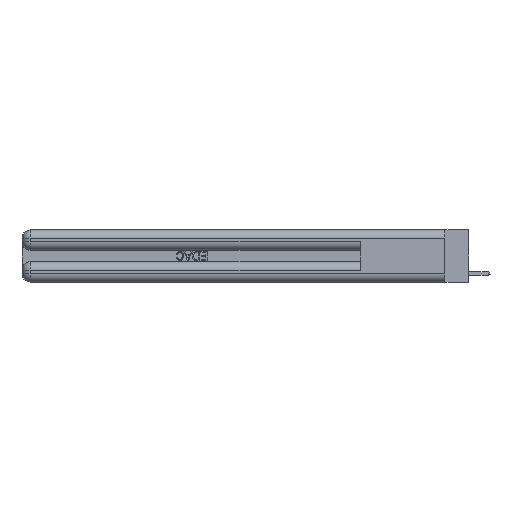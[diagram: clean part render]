
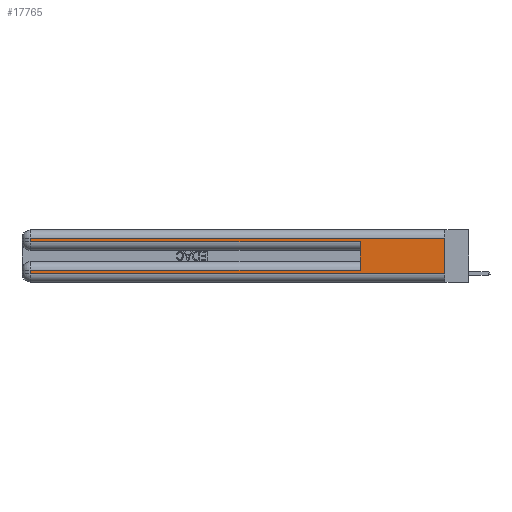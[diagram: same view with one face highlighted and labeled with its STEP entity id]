
A CAD part, left-side view. The second image highlights one B-rep face of the part: STEP entity #17765.
In plain terms, the highlighted planar face has unit normal (-1, 0, 0).
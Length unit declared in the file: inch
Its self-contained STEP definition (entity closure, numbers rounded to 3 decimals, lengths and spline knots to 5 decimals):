
#143 = LINE ( 'NONE', #8147, #11235 ) ;
#225 = CARTESIAN_POINT ( 'NONE',  ( 0., 0.6, 0.285 ) ) ;
#410 = VECTOR ( 'NONE', #3186, 39.37008 ) ;
#485 = ORIENTED_EDGE ( 'NONE', *, *, #15310, .T. ) ;
#815 = FACE_OUTER_BOUND ( 'NONE', #11598, .T. ) ;
#1305 = VECTOR ( 'NONE', #2787, 39.37008 ) ;
#2226 = VERTEX_POINT ( 'NONE', #17701 ) ;
#2661 = LINE ( 'NONE', #22642, #1305 ) ;
#2785 = LINE ( 'NONE', #10650, #12086 ) ;
#2787 = DIRECTION ( 'NONE',  ( 0., -1., 0. ) ) ;
#2983 = VECTOR ( 'NONE', #5240, 39.37008 ) ;
#3186 = DIRECTION ( 'NONE',  ( 0., 0., -1. ) ) ;
#4068 = EDGE_CURVE ( 'NONE', #6127, #8896, #14052, .T. ) ;
#4122 = DIRECTION ( 'NONE',  ( 0., 1., 0. ) ) ;
#4243 = CARTESIAN_POINT ( 'NONE',  ( 0., 0., 0.31 ) ) ;
#4830 = ORIENTED_EDGE ( 'NONE', *, *, #20002, .T. ) ;
#5128 = ORIENTED_EDGE ( 'NONE', *, *, #17338, .F. ) ;
#5240 = DIRECTION ( 'NONE',  ( 0., 0., -1. ) ) ;
#5524 = VECTOR ( 'NONE', #18085, 39.37008 ) ;
#5621 = LINE ( 'NONE', #20860, #410 ) ;
#6036 = CARTESIAN_POINT ( 'NONE',  ( 0., 0.6, 0.085 ) ) ;
#6127 = VERTEX_POINT ( 'NONE', #23041 ) ;
#7196 = ORIENTED_EDGE ( 'NONE', *, *, #24441, .T. ) ;
#7401 = EDGE_CURVE ( 'NONE', #18506, #24398, #5621, .T. ) ;
#8019 = LINE ( 'NONE', #10084, #10055 ) ;
#8147 = CARTESIAN_POINT ( 'NONE',  ( 0., 0., 0.085 ) ) ;
#8896 = VERTEX_POINT ( 'NONE', #18223 ) ;
#9174 = ORIENTED_EDGE ( 'NONE', *, *, #7401, .T. ) ;
#9754 = ORIENTED_EDGE ( 'NONE', *, *, #22672, .F. ) ;
#10055 = VECTOR ( 'NONE', #20135, 39.37008 ) ;
#10084 = CARTESIAN_POINT ( 'NONE',  ( 0., 0.6, 0.145 ) ) ;
#10121 = VECTOR ( 'NONE', #4122, 39.37008 ) ;
#10331 = CARTESIAN_POINT ( 'NONE',  ( 0., 2.94, 0.37 ) ) ;
#10650 = CARTESIAN_POINT ( 'NONE',  ( 0., 0., 0.06 ) ) ;
#10748 = DIRECTION ( 'NONE',  ( 0., 0., -1. ) ) ;
#11235 = VECTOR ( 'NONE', #22086, 39.37008 ) ;
#11598 = EDGE_LOOP ( 'NONE', ( #5128, #17140, #7196, #4830, #9754, #485, #9174, #25451 ) ) ;
#12086 = VECTOR ( 'NONE', #18402, 39.37008 ) ;
#12279 = LINE ( 'NONE', #10331, #5524 ) ;
#12396 = CARTESIAN_POINT ( 'NONE',  ( 0., 2.94, 0.06 ) ) ;
#14052 = LINE ( 'NONE', #4243, #10121 ) ;
#14128 = AXIS2_PLACEMENT_3D ( 'NONE', #22122, #24053, #10748 ) ;
#15310 = EDGE_CURVE ( 'NONE', #18650, #18506, #143, .T. ) ;
#17140 = ORIENTED_EDGE ( 'NONE', *, *, #4068, .T. ) ;
#17338 = EDGE_CURVE ( 'NONE', #6127, #21455, #17361, .T. ) ;
#17361 = LINE ( 'NONE', #23294, #2983 ) ;
#17701 = CARTESIAN_POINT ( 'NONE',  ( 0., 2.94, 0.285 ) ) ;
#17765 = ADVANCED_FACE ( 'NONE', ( #815 ), #20552, .F. ) ;
#18085 = DIRECTION ( 'NONE',  ( 0., 0., -1. ) ) ;
#18223 = CARTESIAN_POINT ( 'NONE',  ( 0., 2.94, 0.31 ) ) ;
#18402 = DIRECTION ( 'NONE',  ( 0., -1., 0. ) ) ;
#18506 = VERTEX_POINT ( 'NONE', #24510 ) ;
#18650 = VERTEX_POINT ( 'NONE', #6036 ) ;
#18956 = VERTEX_POINT ( 'NONE', #225 ) ;
#20002 = EDGE_CURVE ( 'NONE', #2226, #18956, #2661, .T. ) ;
#20135 = DIRECTION ( 'NONE',  ( 0., 0., 1. ) ) ;
#20552 = PLANE ( 'NONE',  #14128 ) ;
#20860 = CARTESIAN_POINT ( 'NONE',  ( 0., 2.94, 0.37 ) ) ;
#21455 = VERTEX_POINT ( 'NONE', #24238 ) ;
#21811 = EDGE_CURVE ( 'NONE', #24398, #21455, #2785, .T. ) ;
#22086 = DIRECTION ( 'NONE',  ( 0., 1., 0. ) ) ;
#22122 = CARTESIAN_POINT ( 'NONE',  ( 0., 0., 0.37 ) ) ;
#22642 = CARTESIAN_POINT ( 'NONE',  ( 0., 0., 0.285 ) ) ;
#22672 = EDGE_CURVE ( 'NONE', #18650, #18956, #8019, .T. ) ;
#23041 = CARTESIAN_POINT ( 'NONE',  ( 0., 0., 0.31 ) ) ;
#23294 = CARTESIAN_POINT ( 'NONE',  ( 0., 0., 0.37 ) ) ;
#24053 = DIRECTION ( 'NONE',  ( 1., 0., 0. ) ) ;
#24238 = CARTESIAN_POINT ( 'NONE',  ( 0., 0., 0.06 ) ) ;
#24398 = VERTEX_POINT ( 'NONE', #12396 ) ;
#24441 = EDGE_CURVE ( 'NONE', #8896, #2226, #12279, .T. ) ;
#24510 = CARTESIAN_POINT ( 'NONE',  ( 0., 2.94, 0.085 ) ) ;
#25451 = ORIENTED_EDGE ( 'NONE', *, *, #21811, .T. ) ;
